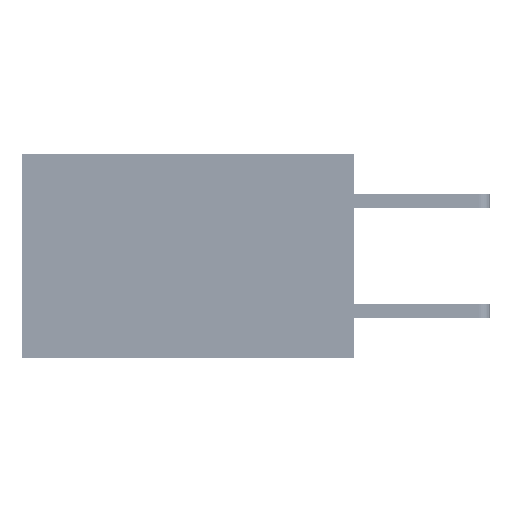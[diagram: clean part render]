
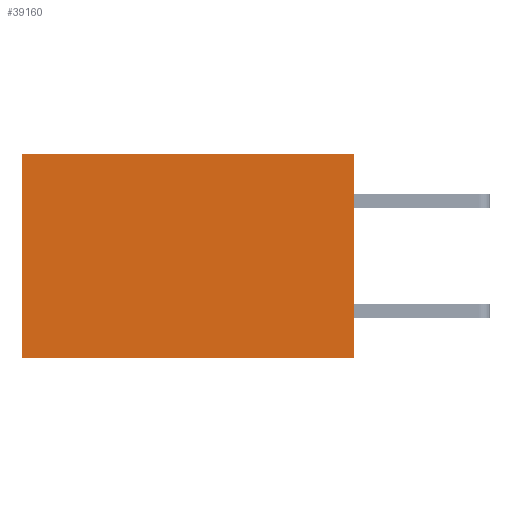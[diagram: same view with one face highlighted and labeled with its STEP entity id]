
A CAD part, left-side view. The second image highlights one B-rep face of the part: STEP entity #39160.
In plain terms, the highlighted planar face has unit normal (-1, 0, 0).
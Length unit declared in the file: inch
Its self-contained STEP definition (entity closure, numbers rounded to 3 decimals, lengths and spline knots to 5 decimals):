
#2017 = EDGE_LOOP ( 'NONE', ( #21631, #34799, #31657, #18218 ) ) ;
#4483 = VECTOR ( 'NONE', #34921, 39.37008 ) ;
#6438 = CARTESIAN_POINT ( 'NONE',  ( 0.2875, 0., 0. ) ) ;
#7249 = LINE ( 'NONE', #42409, #48525 ) ;
#7367 = CARTESIAN_POINT ( 'NONE',  ( 0.2875, 0.6, 0. ) ) ;
#8180 = CARTESIAN_POINT ( 'NONE',  ( 0.2875, 0., -0.37 ) ) ;
#8652 = VERTEX_POINT ( 'NONE', #36123 ) ;
#10211 = LINE ( 'NONE', #6438, #12651 ) ;
#12651 = VECTOR ( 'NONE', #48918, 39.37008 ) ;
#13581 = VERTEX_POINT ( 'NONE', #34332 ) ;
#13943 = AXIS2_PLACEMENT_3D ( 'NONE', #31880, #24531, #47105 ) ;
#16277 = VERTEX_POINT ( 'NONE', #35188 ) ;
#18218 = ORIENTED_EDGE ( 'NONE', *, *, #25252, .T. ) ;
#19168 = EDGE_CURVE ( 'NONE', #8652, #34298, #27241, .T. ) ;
#21631 = ORIENTED_EDGE ( 'NONE', *, *, #32249, .T. ) ;
#23025 = DIRECTION ( 'NONE',  ( 0., 1., 0. ) ) ;
#24207 = PLANE ( 'NONE',  #13943 ) ;
#24531 = DIRECTION ( 'NONE',  ( 1., 0., 0. ) ) ;
#24631 = FACE_OUTER_BOUND ( 'NONE', #2017, .T. ) ;
#25252 = EDGE_CURVE ( 'NONE', #16277, #13581, #7249, .T. ) ;
#27241 = LINE ( 'NONE', #8180, #4483 ) ;
#29810 = VECTOR ( 'NONE', #34109, 39.37008 ) ;
#30498 = EDGE_CURVE ( 'NONE', #16277, #8652, #10211, .T. ) ;
#31657 = ORIENTED_EDGE ( 'NONE', *, *, #30498, .F. ) ;
#31880 = CARTESIAN_POINT ( 'NONE',  ( 0.2875, 0., 0. ) ) ;
#32249 = EDGE_CURVE ( 'NONE', #13581, #34298, #40533, .T. ) ;
#34109 = DIRECTION ( 'NONE',  ( 0., 0., -1. ) ) ;
#34298 = VERTEX_POINT ( 'NONE', #44307 ) ;
#34332 = CARTESIAN_POINT ( 'NONE',  ( 0.2875, 0.6, 0. ) ) ;
#34799 = ORIENTED_EDGE ( 'NONE', *, *, #19168, .F. ) ;
#34921 = DIRECTION ( 'NONE',  ( 0., 1., 0. ) ) ;
#35188 = CARTESIAN_POINT ( 'NONE',  ( 0.2875, 0., 0. ) ) ;
#36123 = CARTESIAN_POINT ( 'NONE',  ( 0.2875, 0., -0.37 ) ) ;
#39160 = ADVANCED_FACE ( 'NONE', ( #24631 ), #24207, .F. ) ;
#40533 = LINE ( 'NONE', #7367, #29810 ) ;
#42409 = CARTESIAN_POINT ( 'NONE',  ( 0.2875, 0., 0. ) ) ;
#44307 = CARTESIAN_POINT ( 'NONE',  ( 0.2875, 0.6, -0.37 ) ) ;
#47105 = DIRECTION ( 'NONE',  ( 0., 0., -1. ) ) ;
#48525 = VECTOR ( 'NONE', #23025, 39.37008 ) ;
#48918 = DIRECTION ( 'NONE',  ( 0., 0., -1. ) ) ;
